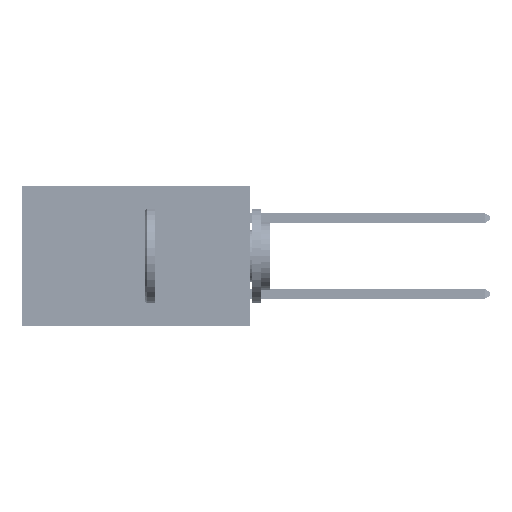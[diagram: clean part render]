
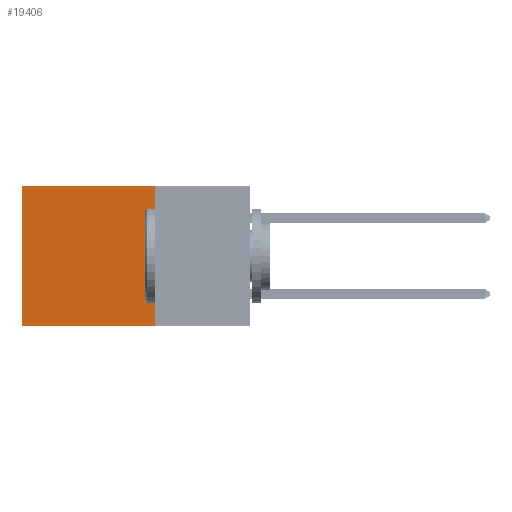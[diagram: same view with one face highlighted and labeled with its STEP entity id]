
A CAD part, left-side view. The second image highlights one B-rep face of the part: STEP entity #19406.
In plain terms, the highlighted planar face has unit normal (-1, 0, 0).
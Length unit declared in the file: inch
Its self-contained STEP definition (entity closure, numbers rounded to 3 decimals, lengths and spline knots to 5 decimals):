
#705 = VERTEX_POINT ( 'NONE', #40327 ) ;
#1559 = CARTESIAN_POINT ( 'NONE',  ( 0.2875, 0.6, 0. ) ) ;
#4773 = PLANE ( 'NONE',  #18866 ) ;
#5838 = CARTESIAN_POINT ( 'NONE',  ( 0.2875, 0.25, -0.37 ) ) ;
#6402 = VECTOR ( 'NONE', #28303, 39.37008 ) ;
#6888 = DIRECTION ( 'NONE',  ( 0., 1., 0. ) ) ;
#14565 = VERTEX_POINT ( 'NONE', #5838 ) ;
#14874 = CARTESIAN_POINT ( 'NONE',  ( 0.2875, 0.25, -0.37 ) ) ;
#15361 = VECTOR ( 'NONE', #31558, 39.37008 ) ;
#15892 = EDGE_CURVE ( 'NONE', #18456, #705, #45006, .T. ) ;
#18308 = CARTESIAN_POINT ( 'NONE',  ( 0.2875, 0.25, 0. ) ) ;
#18456 = VERTEX_POINT ( 'NONE', #44265 ) ;
#18492 = LINE ( 'NONE', #39490, #27323 ) ;
#18866 = AXIS2_PLACEMENT_3D ( 'NONE', #31158, #30817, #42445 ) ;
#19406 = ADVANCED_FACE ( 'NONE', ( #48659 ), #4773, .F. ) ;
#20883 = ORIENTED_EDGE ( 'NONE', *, *, #20973, .F. ) ;
#20973 = EDGE_CURVE ( 'NONE', #14565, #705, #31213, .T. ) ;
#21170 = VECTOR ( 'NONE', #6888, 39.37008 ) ;
#25435 = LINE ( 'NONE', #47225, #15361 ) ;
#27089 = EDGE_LOOP ( 'NONE', ( #39720, #20883, #31977, #32615 ) ) ;
#27323 = VECTOR ( 'NONE', #43314, 39.37008 ) ;
#28303 = DIRECTION ( 'NONE',  ( 0., 0., -1. ) ) ;
#30817 = DIRECTION ( 'NONE',  ( 1., 0., 0. ) ) ;
#31158 = CARTESIAN_POINT ( 'NONE',  ( 0.2875, 0.25, 0. ) ) ;
#31213 = LINE ( 'NONE', #14874, #21170 ) ;
#31558 = DIRECTION ( 'NONE',  ( 0., 1., 0. ) ) ;
#31977 = ORIENTED_EDGE ( 'NONE', *, *, #35933, .F. ) ;
#32615 = ORIENTED_EDGE ( 'NONE', *, *, #40660, .T. ) ;
#34247 = VERTEX_POINT ( 'NONE', #18308 ) ;
#35933 = EDGE_CURVE ( 'NONE', #34247, #14565, #18492, .T. ) ;
#39490 = CARTESIAN_POINT ( 'NONE',  ( 0.2875, 0.25, 0. ) ) ;
#39720 = ORIENTED_EDGE ( 'NONE', *, *, #15892, .T. ) ;
#40327 = CARTESIAN_POINT ( 'NONE',  ( 0.2875, 0.6, -0.37 ) ) ;
#40660 = EDGE_CURVE ( 'NONE', #34247, #18456, #25435, .T. ) ;
#42445 = DIRECTION ( 'NONE',  ( 0., 0., -1. ) ) ;
#43314 = DIRECTION ( 'NONE',  ( 0., 0., -1. ) ) ;
#44265 = CARTESIAN_POINT ( 'NONE',  ( 0.2875, 0.6, 0. ) ) ;
#45006 = LINE ( 'NONE', #1559, #6402 ) ;
#47225 = CARTESIAN_POINT ( 'NONE',  ( 0.2875, 0.25, 0. ) ) ;
#48659 = FACE_OUTER_BOUND ( 'NONE', #27089, .T. ) ;
